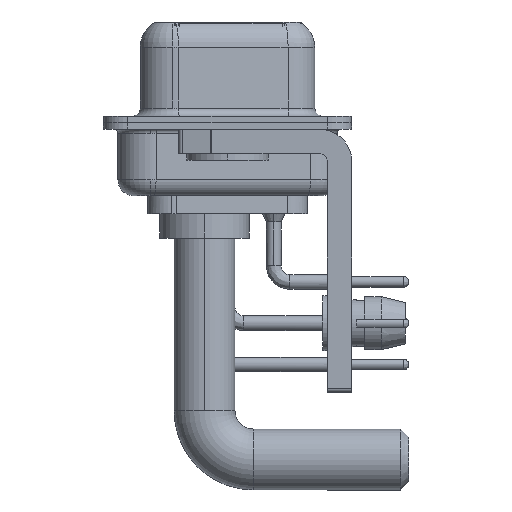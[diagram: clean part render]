
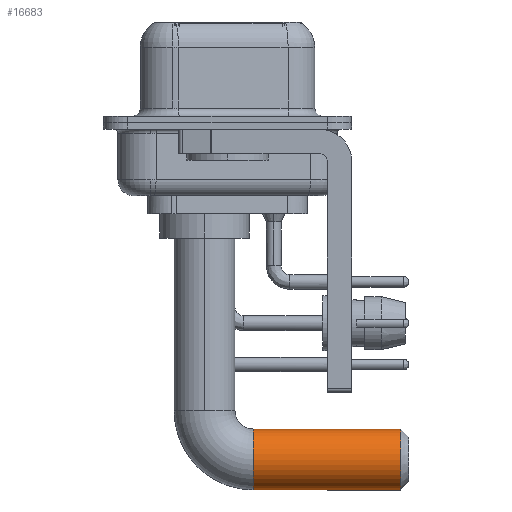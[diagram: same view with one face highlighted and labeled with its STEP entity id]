
A CAD part, left-side view. The second image highlights one B-rep face of the part: STEP entity #16683.
In plain terms, the highlighted cylindrical face has radius 1.875 mm (diameter 3.75 mm), a partial arc.
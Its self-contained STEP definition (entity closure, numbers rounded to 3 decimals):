
#431 = CIRCLE ( 'NONE', #10180, 1.875 ) ;
#719 = VECTOR ( 'NONE', #15065, 1000. ) ;
#1072 = ORIENTED_EDGE ( 'NONE', *, *, #29927, .F. ) ;
#1377 = CYLINDRICAL_SURFACE ( 'NONE', #12749, 1.875 ) ;
#1567 = LINE ( 'NONE', #18758, #18252 ) ;
#1574 = EDGE_CURVE ( 'NONE', #6940, #19583, #17289, .T. ) ;
#2737 = EDGE_CURVE ( 'NONE', #25325, #15648, #431, .T. ) ;
#4350 = CARTESIAN_POINT ( 'NONE',  ( 0., -12.07, -13.63 ) ) ;
#5600 = DIRECTION ( 'NONE',  ( -1., 0., 0. ) ) ;
#6821 = DIRECTION ( 'NONE',  ( 0., 0., -1. ) ) ;
#6902 = DIRECTION ( 'NONE',  ( 0., 1., 0. ) ) ;
#6940 = VERTEX_POINT ( 'NONE', #29385 ) ;
#7888 = EDGE_LOOP ( 'NONE', ( #1072, #15189, #27059, #31628 ) ) ;
#9314 = DIRECTION ( 'NONE',  ( 0., 0., -1. ) ) ;
#10180 = AXIS2_PLACEMENT_3D ( 'NONE', #20371, #16023, #5600 ) ;
#10264 = CARTESIAN_POINT ( 'NONE',  ( 0., -3., -15.505 ) ) ;
#12749 = AXIS2_PLACEMENT_3D ( 'NONE', #31061, #19201, #6821 ) ;
#12804 = EDGE_CURVE ( 'NONE', #15648, #6940, #1567, .T. ) ;
#14720 = AXIS2_PLACEMENT_3D ( 'NONE', #4350, #6902, #9314 ) ;
#15065 = DIRECTION ( 'NONE',  ( 0., -1., 0. ) ) ;
#15189 = ORIENTED_EDGE ( 'NONE', *, *, #2737, .T. ) ;
#15648 = VERTEX_POINT ( 'NONE', #10264 ) ;
#16023 = DIRECTION ( 'NONE',  ( 0., -1., 0. ) ) ;
#16622 = CARTESIAN_POINT ( 'NONE',  ( 0., -12.07, -11.755 ) ) ;
#16683 = ADVANCED_FACE ( 'NONE', ( #23383 ), #1377, .T. ) ;
#17289 = CIRCLE ( 'NONE', #14720, 1.875 ) ;
#17294 = CARTESIAN_POINT ( 'NONE',  ( 0., -3., -11.755 ) ) ;
#17485 = LINE ( 'NONE', #22128, #719 ) ;
#18252 = VECTOR ( 'NONE', #30622, 1000. ) ;
#18758 = CARTESIAN_POINT ( 'NONE',  ( 0., -3., -15.505 ) ) ;
#19201 = DIRECTION ( 'NONE',  ( 0., -1., 0. ) ) ;
#19583 = VERTEX_POINT ( 'NONE', #16622 ) ;
#20371 = CARTESIAN_POINT ( 'NONE',  ( 0., -3., -13.63 ) ) ;
#22128 = CARTESIAN_POINT ( 'NONE',  ( 0., -3., -11.755 ) ) ;
#23383 = FACE_OUTER_BOUND ( 'NONE', #7888, .T. ) ;
#25325 = VERTEX_POINT ( 'NONE', #17294 ) ;
#27059 = ORIENTED_EDGE ( 'NONE', *, *, #12804, .T. ) ;
#29385 = CARTESIAN_POINT ( 'NONE',  ( 0., -12.07, -15.505 ) ) ;
#29927 = EDGE_CURVE ( 'NONE', #25325, #19583, #17485, .T. ) ;
#30622 = DIRECTION ( 'NONE',  ( 0., -1., 0. ) ) ;
#31061 = CARTESIAN_POINT ( 'NONE',  ( 0., -3., -13.63 ) ) ;
#31628 = ORIENTED_EDGE ( 'NONE', *, *, #1574, .T. ) ;
